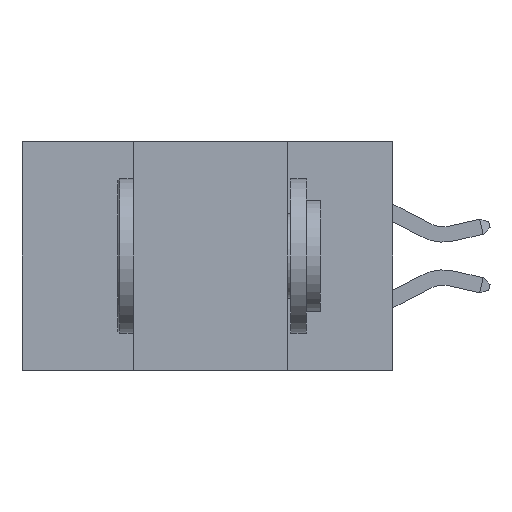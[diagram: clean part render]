
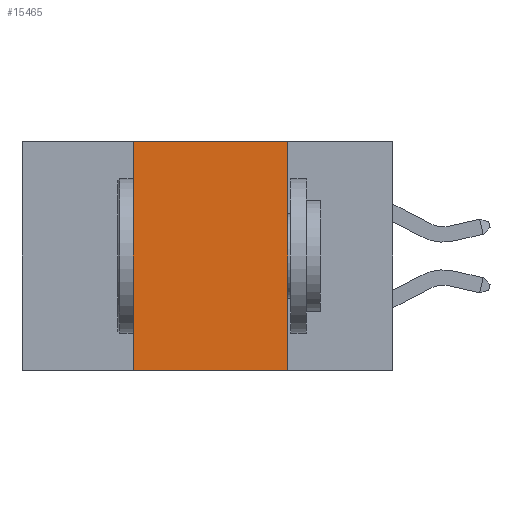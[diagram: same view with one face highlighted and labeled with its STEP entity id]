
A CAD part, left-side view. The second image highlights one B-rep face of the part: STEP entity #15465.
In plain terms, the highlighted planar face has unit normal (-1, 0, 0).
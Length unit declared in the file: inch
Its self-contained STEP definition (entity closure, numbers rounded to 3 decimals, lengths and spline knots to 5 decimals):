
#39 = DIRECTION ( 'NONE',  ( 0., 0., -1. ) ) ;
#1052 = VECTOR ( 'NONE', #12291, 39.37008 ) ;
#2696 = ORIENTED_EDGE ( 'NONE', *, *, #6342, .T. ) ;
#2833 = VERTEX_POINT ( 'NONE', #10075 ) ;
#3119 = LINE ( 'NONE', #18346, #9531 ) ;
#5005 = LINE ( 'NONE', #11948, #12296 ) ;
#5269 = FACE_OUTER_BOUND ( 'NONE', #5791, .T. ) ;
#5310 = DIRECTION ( 'NONE',  ( 0., -1., 0. ) ) ;
#5758 = ORIENTED_EDGE ( 'NONE', *, *, #12581, .F. ) ;
#5791 = EDGE_LOOP ( 'NONE', ( #5758, #9576, #13929, #2696 ) ) ;
#6342 = EDGE_CURVE ( 'NONE', #2833, #11043, #3119, .T. ) ;
#6497 = LINE ( 'NONE', #8970, #10791 ) ;
#6919 = DIRECTION ( 'NONE',  ( 1., 0., 0. ) ) ;
#7075 = CARTESIAN_POINT ( 'NONE',  ( 0., 0.17, -0.37 ) ) ;
#7238 = VERTEX_POINT ( 'NONE', #13290 ) ;
#7457 = CARTESIAN_POINT ( 'NONE',  ( 0., 0.6, 0. ) ) ;
#8970 = CARTESIAN_POINT ( 'NONE',  ( 0., 0.17, 0. ) ) ;
#9436 = EDGE_CURVE ( 'NONE', #7238, #11335, #12857, .T. ) ;
#9531 = VECTOR ( 'NONE', #5310, 39.37008 ) ;
#9576 = ORIENTED_EDGE ( 'NONE', *, *, #9436, .F. ) ;
#10075 = CARTESIAN_POINT ( 'NONE',  ( 0., 0.42, -0.37 ) ) ;
#10354 = DIRECTION ( 'NONE',  ( 0., 0., -1. ) ) ;
#10791 = VECTOR ( 'NONE', #39, 39.37008 ) ;
#10810 = CARTESIAN_POINT ( 'NONE',  ( 0., 0.6, 0. ) ) ;
#11043 = VERTEX_POINT ( 'NONE', #7075 ) ;
#11335 = VERTEX_POINT ( 'NONE', #13537 ) ;
#11948 = CARTESIAN_POINT ( 'NONE',  ( 0., 0.42, 0. ) ) ;
#12291 = DIRECTION ( 'NONE',  ( 0., -1., 0. ) ) ;
#12296 = VECTOR ( 'NONE', #13409, 39.37008 ) ;
#12581 = EDGE_CURVE ( 'NONE', #11335, #11043, #6497, .T. ) ;
#12857 = LINE ( 'NONE', #10810, #1052 ) ;
#13290 = CARTESIAN_POINT ( 'NONE',  ( 0., 0.42, 0. ) ) ;
#13409 = DIRECTION ( 'NONE',  ( 0., 0., 1. ) ) ;
#13537 = CARTESIAN_POINT ( 'NONE',  ( 0., 0.17, 0. ) ) ;
#13929 = ORIENTED_EDGE ( 'NONE', *, *, #16133, .F. ) ;
#15465 = ADVANCED_FACE ( 'NONE', ( #5269 ), #16214, .F. ) ;
#16133 = EDGE_CURVE ( 'NONE', #2833, #7238, #5005, .T. ) ;
#16214 = PLANE ( 'NONE',  #16808 ) ;
#16808 = AXIS2_PLACEMENT_3D ( 'NONE', #7457, #6919, #10354 ) ;
#18346 = CARTESIAN_POINT ( 'NONE',  ( 0., 0.6, -0.37 ) ) ;
